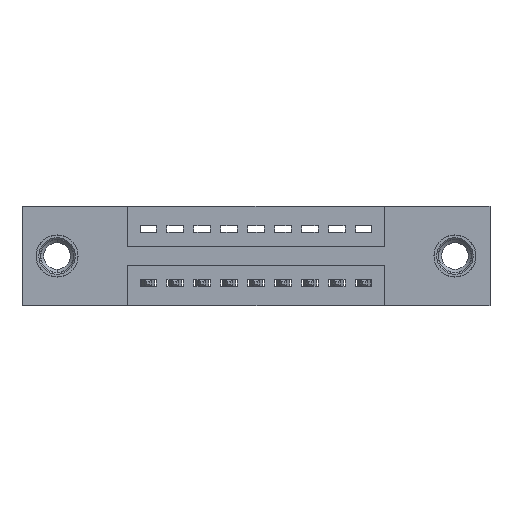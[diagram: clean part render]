
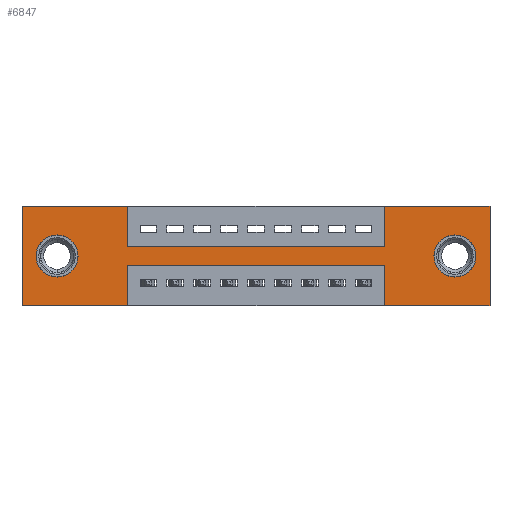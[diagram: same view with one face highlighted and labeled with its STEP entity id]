
A CAD part, front view. The second image highlights one B-rep face of the part: STEP entity #6847.
In plain terms, the highlighted planar face has unit normal (0, -1, 0).
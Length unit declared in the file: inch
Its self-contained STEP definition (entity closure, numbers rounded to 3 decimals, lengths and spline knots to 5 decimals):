
#79 = LINE ( 'NONE', #5805, #5200 ) ;
#89 = FACE_BOUND ( 'NONE', #4199, .T. ) ;
#129 = VECTOR ( 'NONE', #7946, 39.37008 ) ;
#330 = ORIENTED_EDGE ( 'NONE', *, *, #3392, .T. ) ;
#542 = CARTESIAN_POINT ( 'NONE',  ( 1.3425, 0., -0.22 ) ) ;
#560 = DIRECTION ( 'NONE',  ( 0., 0., -1. ) ) ;
#757 = VECTOR ( 'NONE', #4833, 39.37008 ) ;
#805 = EDGE_CURVE ( 'NONE', #10871, #8285, #79, .T. ) ;
#964 = CARTESIAN_POINT ( 'NONE',  ( 0., 0., 0. ) ) ;
#1232 = VERTEX_POINT ( 'NONE', #10435 ) ;
#1543 = LINE ( 'NONE', #4518, #6958 ) ;
#1569 = DIRECTION ( 'NONE',  ( 0., 0., 1. ) ) ;
#1622 = DIRECTION ( 'NONE',  ( 0., 1., 0. ) ) ;
#1710 = EDGE_LOOP ( 'NONE', ( #10973, #3426 ) ) ;
#1750 = CARTESIAN_POINT ( 'NONE',  ( 1.605, 0., -0.185 ) ) ;
#1809 = ORIENTED_EDGE ( 'NONE', *, *, #5382, .T. ) ;
#1933 = CARTESIAN_POINT ( 'NONE',  ( 1.735, 0., -0.37 ) ) ;
#2242 = CARTESIAN_POINT ( 'NONE',  ( 1.3425, 0., -0.15 ) ) ;
#2290 = VERTEX_POINT ( 'NONE', #8304 ) ;
#2344 = PLANE ( 'NONE',  #9518 ) ;
#2436 = EDGE_CURVE ( 'NONE', #2290, #7073, #7720, .T. ) ;
#2501 = CARTESIAN_POINT ( 'NONE',  ( 0., 0., -0.37 ) ) ;
#2618 = AXIS2_PLACEMENT_3D ( 'NONE', #7284, #5259, #1569 ) ;
#2631 = EDGE_CURVE ( 'NONE', #7073, #2290, #9538, .T. ) ;
#2653 = EDGE_CURVE ( 'NONE', #1232, #12082, #12348, .T. ) ;
#2682 = LINE ( 'NONE', #6988, #10826 ) ;
#2694 = ORIENTED_EDGE ( 'NONE', *, *, #8472, .F. ) ;
#2750 = ORIENTED_EDGE ( 'NONE', *, *, #2653, .F. ) ;
#2826 = EDGE_CURVE ( 'NONE', #9805, #6673, #1543, .T. ) ;
#2914 = EDGE_LOOP ( 'NONE', ( #11834, #4665, #7453, #8393, #2750, #10708, #7622, #3798, #6545, #4799, #4439, #2694 ) ) ;
#3254 = LINE ( 'NONE', #2501, #9726 ) ;
#3392 = EDGE_CURVE ( 'NONE', #8608, #9223, #11604, .T. ) ;
#3426 = ORIENTED_EDGE ( 'NONE', *, *, #2436, .T. ) ;
#3464 = DIRECTION ( 'NONE',  ( 1., 0., 0. ) ) ;
#3502 = VERTEX_POINT ( 'NONE', #9971 ) ;
#3534 = AXIS2_PLACEMENT_3D ( 'NONE', #1750, #9361, #8480 ) ;
#3577 = VECTOR ( 'NONE', #3464, 39.37008 ) ;
#3601 = DIRECTION ( 'NONE',  ( 0., 0., -1. ) ) ;
#3773 = DIRECTION ( 'NONE',  ( 1., 0., 0. ) ) ;
#3798 = ORIENTED_EDGE ( 'NONE', *, *, #11998, .F. ) ;
#3829 = CARTESIAN_POINT ( 'NONE',  ( 0.3925, 0., -0.15 ) ) ;
#4045 = DIRECTION ( 'NONE',  ( 0., 0., -1. ) ) ;
#4199 = EDGE_LOOP ( 'NONE', ( #1809, #330 ) ) ;
#4331 = EDGE_CURVE ( 'NONE', #12082, #12244, #10088, .T. ) ;
#4439 = ORIENTED_EDGE ( 'NONE', *, *, #805, .F. ) ;
#4466 = CARTESIAN_POINT ( 'NONE',  ( 0.3925, 0., 0. ) ) ;
#4518 = CARTESIAN_POINT ( 'NONE',  ( 0.3925, 0., 0. ) ) ;
#4618 = EDGE_CURVE ( 'NONE', #9799, #5859, #10389, .T. ) ;
#4665 = ORIENTED_EDGE ( 'NONE', *, *, #4618, .F. ) ;
#4778 = CARTESIAN_POINT ( 'NONE',  ( 1.3425, 0., -0.37 ) ) ;
#4799 = ORIENTED_EDGE ( 'NONE', *, *, #7441, .F. ) ;
#4833 = DIRECTION ( 'NONE',  ( 1., 0., 0. ) ) ;
#4952 = VECTOR ( 'NONE', #6173, 39.37008 ) ;
#5200 = VECTOR ( 'NONE', #5377, 39.37008 ) ;
#5259 = DIRECTION ( 'NONE',  ( 0., 1., 0. ) ) ;
#5298 = CARTESIAN_POINT ( 'NONE',  ( 0., 0., 0. ) ) ;
#5330 = EDGE_CURVE ( 'NONE', #5859, #3502, #2682, .T. ) ;
#5377 = DIRECTION ( 'NONE',  ( 0., 0., 1. ) ) ;
#5382 = EDGE_CURVE ( 'NONE', #9223, #8608, #7965, .T. ) ;
#5708 = CARTESIAN_POINT ( 'NONE',  ( 0.13, 0., -0.107 ) ) ;
#5805 = CARTESIAN_POINT ( 'NONE',  ( 0., 0., 0. ) ) ;
#5829 = EDGE_CURVE ( 'NONE', #12244, #9799, #11710, .T. ) ;
#5859 = VERTEX_POINT ( 'NONE', #7388 ) ;
#5989 = DIRECTION ( 'NONE',  ( 0., 0., 1. ) ) ;
#6142 = CARTESIAN_POINT ( 'NONE',  ( 0., 0., -0.37 ) ) ;
#6173 = DIRECTION ( 'NONE',  ( -1., 0., 0. ) ) ;
#6226 = CARTESIAN_POINT ( 'NONE',  ( 0., 0., 0. ) ) ;
#6545 = ORIENTED_EDGE ( 'NONE', *, *, #2826, .F. ) ;
#6673 = VERTEX_POINT ( 'NONE', #8844 ) ;
#6766 = AXIS2_PLACEMENT_3D ( 'NONE', #11933, #9061, #10118 ) ;
#6847 = ADVANCED_FACE ( 'NONE', ( #9133, #89, #11678 ), #2344, .T. ) ;
#6895 = AXIS2_PLACEMENT_3D ( 'NONE', #7258, #1622, #560 ) ;
#6921 = CARTESIAN_POINT ( 'NONE',  ( 1.3425, 0., 0. ) ) ;
#6925 = LINE ( 'NONE', #3829, #757 ) ;
#6958 = VECTOR ( 'NONE', #3601, 39.37008 ) ;
#6969 = VECTOR ( 'NONE', #7392, 39.37008 ) ;
#6988 = CARTESIAN_POINT ( 'NONE',  ( 0.3925, 0., -0.37 ) ) ;
#7073 = VERTEX_POINT ( 'NONE', #10065 ) ;
#7098 = CARTESIAN_POINT ( 'NONE',  ( 0.3925, 0., -0.22 ) ) ;
#7104 = DIRECTION ( 'NONE',  ( 0., 0., -1. ) ) ;
#7193 = DIRECTION ( 'NONE',  ( 0., -1., 0. ) ) ;
#7258 = CARTESIAN_POINT ( 'NONE',  ( 1.605, 0., -0.185 ) ) ;
#7284 = CARTESIAN_POINT ( 'NONE',  ( 0.13, 0., -0.185 ) ) ;
#7388 = CARTESIAN_POINT ( 'NONE',  ( 0.3925, 0., -0.22 ) ) ;
#7392 = DIRECTION ( 'NONE',  ( 0., 0., -1. ) ) ;
#7441 = EDGE_CURVE ( 'NONE', #8285, #9805, #10216, .T. ) ;
#7453 = ORIENTED_EDGE ( 'NONE', *, *, #5829, .F. ) ;
#7622 = ORIENTED_EDGE ( 'NONE', *, *, #7668, .F. ) ;
#7668 = EDGE_CURVE ( 'NONE', #9135, #11065, #7772, .T. ) ;
#7720 = CIRCLE ( 'NONE', #3534, 0.078 ) ;
#7772 = LINE ( 'NONE', #8133, #10497 ) ;
#7880 = EDGE_CURVE ( 'NONE', #11065, #1232, #9122, .T. ) ;
#7946 = DIRECTION ( 'NONE',  ( -1., 0., 0. ) ) ;
#7965 = CIRCLE ( 'NONE', #6766, 0.078 ) ;
#8133 = CARTESIAN_POINT ( 'NONE',  ( 1.3425, 0., 0. ) ) ;
#8183 = DIRECTION ( 'NONE',  ( -1., 0., 0. ) ) ;
#8285 = VERTEX_POINT ( 'NONE', #6226 ) ;
#8304 = CARTESIAN_POINT ( 'NONE',  ( 1.605, 0., -0.263 ) ) ;
#8393 = ORIENTED_EDGE ( 'NONE', *, *, #4331, .F. ) ;
#8472 = EDGE_CURVE ( 'NONE', #3502, #10871, #3254, .T. ) ;
#8480 = DIRECTION ( 'NONE',  ( 0., 0., -1. ) ) ;
#8539 = VECTOR ( 'NONE', #3773, 39.37008 ) ;
#8608 = VERTEX_POINT ( 'NONE', #10310 ) ;
#8844 = CARTESIAN_POINT ( 'NONE',  ( 0.3925, 0., -0.15 ) ) ;
#9061 = DIRECTION ( 'NONE',  ( 0., 1., 0. ) ) ;
#9122 = LINE ( 'NONE', #5298, #3577 ) ;
#9133 = FACE_BOUND ( 'NONE', #1710, .T. ) ;
#9135 = VERTEX_POINT ( 'NONE', #2242 ) ;
#9223 = VERTEX_POINT ( 'NONE', #5708 ) ;
#9361 = DIRECTION ( 'NONE',  ( 0., 1., 0. ) ) ;
#9518 = AXIS2_PLACEMENT_3D ( 'NONE', #6142, #7193, #7104 ) ;
#9538 = CIRCLE ( 'NONE', #6895, 0.078 ) ;
#9726 = VECTOR ( 'NONE', #8183, 39.37008 ) ;
#9799 = VERTEX_POINT ( 'NONE', #542 ) ;
#9805 = VERTEX_POINT ( 'NONE', #4466 ) ;
#9971 = CARTESIAN_POINT ( 'NONE',  ( 0.3925, 0., -0.37 ) ) ;
#10065 = CARTESIAN_POINT ( 'NONE',  ( 1.605, 0., -0.107 ) ) ;
#10080 = DIRECTION ( 'NONE',  ( 0., 0., 1. ) ) ;
#10088 = LINE ( 'NONE', #11948, #4952 ) ;
#10118 = DIRECTION ( 'NONE',  ( 0., 0., 1. ) ) ;
#10216 = LINE ( 'NONE', #964, #8539 ) ;
#10229 = VECTOR ( 'NONE', #5989, 39.37008 ) ;
#10310 = CARTESIAN_POINT ( 'NONE',  ( 0.13, 0., -0.263 ) ) ;
#10389 = LINE ( 'NONE', #7098, #129 ) ;
#10393 = CARTESIAN_POINT ( 'NONE',  ( 0., 0., -0.37 ) ) ;
#10435 = CARTESIAN_POINT ( 'NONE',  ( 1.735, 0., 0. ) ) ;
#10469 = CARTESIAN_POINT ( 'NONE',  ( 1.3425, 0., -0.37 ) ) ;
#10497 = VECTOR ( 'NONE', #10080, 39.37008 ) ;
#10708 = ORIENTED_EDGE ( 'NONE', *, *, #7880, .F. ) ;
#10826 = VECTOR ( 'NONE', #4045, 39.37008 ) ;
#10871 = VERTEX_POINT ( 'NONE', #10393 ) ;
#10973 = ORIENTED_EDGE ( 'NONE', *, *, #2631, .T. ) ;
#11065 = VERTEX_POINT ( 'NONE', #6921 ) ;
#11604 = CIRCLE ( 'NONE', #2618, 0.078 ) ;
#11678 = FACE_OUTER_BOUND ( 'NONE', #2914, .T. ) ;
#11710 = LINE ( 'NONE', #10469, #10229 ) ;
#11834 = ORIENTED_EDGE ( 'NONE', *, *, #5330, .F. ) ;
#11933 = CARTESIAN_POINT ( 'NONE',  ( 0.13, 0., -0.185 ) ) ;
#11948 = CARTESIAN_POINT ( 'NONE',  ( 0., 0., -0.37 ) ) ;
#11998 = EDGE_CURVE ( 'NONE', #6673, #9135, #6925, .T. ) ;
#12082 = VERTEX_POINT ( 'NONE', #1933 ) ;
#12153 = CARTESIAN_POINT ( 'NONE',  ( 1.735, 0., 0. ) ) ;
#12244 = VERTEX_POINT ( 'NONE', #4778 ) ;
#12348 = LINE ( 'NONE', #12153, #6969 ) ;
